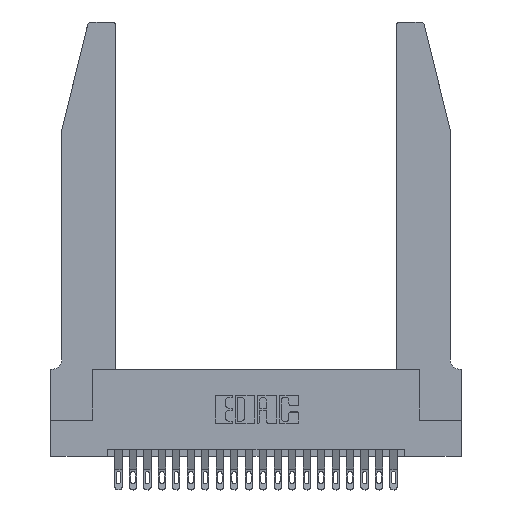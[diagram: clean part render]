
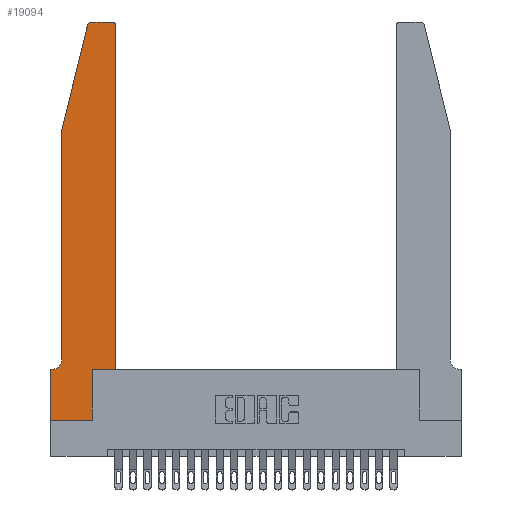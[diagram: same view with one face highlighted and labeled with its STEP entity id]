
A CAD part, top view. The second image highlights one B-rep face of the part: STEP entity #19094.
In plain terms, the highlighted planar face has unit normal (0, 0, 1).
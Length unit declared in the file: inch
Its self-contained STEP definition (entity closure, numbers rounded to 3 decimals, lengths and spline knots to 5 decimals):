
#271 = EDGE_CURVE ( 'NONE', #17309, #3389, #23285, .T. ) ;
#489 = CIRCLE ( 'NONE', #20541, 0.03 ) ;
#499 = DIRECTION ( 'NONE',  ( -0.239, -0.971, 0. ) ) ;
#606 = CARTESIAN_POINT ( 'NONE',  ( 0.4205, 2.72, 0.37 ) ) ;
#1068 = AXIS2_PLACEMENT_3D ( 'NONE', #5403, #18221, #7333 ) ;
#1088 = EDGE_CURVE ( 'NONE', #18876, #5038, #19748, .T. ) ;
#1273 = DIRECTION ( 'NONE',  ( 1., 0., 0. ) ) ;
#1359 = DIRECTION ( 'NONE',  ( 0., -1., 0. ) ) ;
#1726 = VERTEX_POINT ( 'NONE', #6758 ) ;
#1864 = CARTESIAN_POINT ( 'NONE',  ( 0.25487, 2.72718, 0.37 ) ) ;
#1869 = VECTOR ( 'NONE', #23675, 39.37008 ) ;
#1931 = EDGE_CURVE ( 'NONE', #5723, #22449, #6940, .T. ) ;
#2140 = ORIENTED_EDGE ( 'NONE', *, *, #1088, .T. ) ;
#2168 = VERTEX_POINT ( 'NONE', #3895 ) ;
#2270 = CARTESIAN_POINT ( 'NONE',  ( 0., 0.35, 0.37 ) ) ;
#2541 = DIRECTION ( 'NONE',  ( 1., 0., 0. ) ) ;
#2691 = EDGE_CURVE ( 'NONE', #18777, #18876, #12182, .T. ) ;
#3153 = CIRCLE ( 'NONE', #1068, 0.07 ) ;
#3180 = PLANE ( 'NONE',  #20446 ) ;
#3389 = VERTEX_POINT ( 'NONE', #19298 ) ;
#3895 = CARTESIAN_POINT ( 'NONE',  ( 0.0055, 0.35, 0.37 ) ) ;
#4066 = CARTESIAN_POINT ( 'NONE',  ( 0.4205, 2.75, 0.37 ) ) ;
#4377 = CARTESIAN_POINT ( 'NONE',  ( 0.0755, 2., 0.37 ) ) ;
#4488 = VERTEX_POINT ( 'NONE', #22270 ) ;
#4607 = EDGE_CURVE ( 'NONE', #21902, #5723, #18485, .T. ) ;
#4656 = VECTOR ( 'NONE', #5742, 39.37008 ) ;
#5038 = VERTEX_POINT ( 'NONE', #21862 ) ;
#5403 = CARTESIAN_POINT ( 'NONE',  ( 0.0055, 0.42, 0.37 ) ) ;
#5723 = VERTEX_POINT ( 'NONE', #9866 ) ;
#5742 = DIRECTION ( 'NONE',  ( 0., 1., 0. ) ) ;
#5915 = ORIENTED_EDGE ( 'NONE', *, *, #11713, .T. ) ;
#6308 = ORIENTED_EDGE ( 'NONE', *, *, #20932, .T. ) ;
#6758 = CARTESIAN_POINT ( 'NONE',  ( 0.2865, 0.35, 0.37 ) ) ;
#6940 = LINE ( 'NONE', #14252, #1869 ) ;
#7024 = CARTESIAN_POINT ( 'NONE',  ( 0., 0.35, 0.37 ) ) ;
#7093 = CARTESIAN_POINT ( 'NONE',  ( 0.2605, 2.75, 0.37 ) ) ;
#7333 = DIRECTION ( 'NONE',  ( -1., 0., 0. ) ) ;
#7954 = VERTEX_POINT ( 'NONE', #11986 ) ;
#7981 = EDGE_CURVE ( 'NONE', #7954, #4488, #15835, .T. ) ;
#8278 = VECTOR ( 'NONE', #499, 39.37008 ) ;
#8295 = DIRECTION ( 'NONE',  ( 0., 1., 0. ) ) ;
#9137 = CIRCLE ( 'NONE', #20680, 0.03 ) ;
#9436 = EDGE_LOOP ( 'NONE', ( #10798, #17330, #14394, #10636, #5915, #6308, #18889, #2140, #14486, #20805, #21057, #19264 ) ) ;
#9866 = CARTESIAN_POINT ( 'NONE',  ( 0.0755, 2., 0.37 ) ) ;
#10212 = VECTOR ( 'NONE', #17427, 39.37008 ) ;
#10486 = LINE ( 'NONE', #14437, #18902 ) ;
#10636 = ORIENTED_EDGE ( 'NONE', *, *, #1931, .T. ) ;
#10798 = ORIENTED_EDGE ( 'NONE', *, *, #271, .T. ) ;
#11656 = CARTESIAN_POINT ( 'NONE',  ( 0., 0., 0.37 ) ) ;
#11713 = EDGE_CURVE ( 'NONE', #22449, #2168, #3153, .T. ) ;
#11849 = EDGE_CURVE ( 'NONE', #5038, #1726, #19782, .T. ) ;
#11914 = CARTESIAN_POINT ( 'NONE',  ( 0.0755, 0.35, 0.37 ) ) ;
#11986 = CARTESIAN_POINT ( 'NONE',  ( 0.4505, 0.35, 0.37 ) ) ;
#12066 = CARTESIAN_POINT ( 'NONE',  ( 0.4505, 0.35, 0.37 ) ) ;
#12182 = LINE ( 'NONE', #11656, #21630 ) ;
#12587 = DIRECTION ( 'NONE',  ( 0., 0., 1. ) ) ;
#12662 = DIRECTION ( 'NONE',  ( 1., 0., 0. ) ) ;
#13810 = DIRECTION ( 'NONE',  ( 0., 0., 1. ) ) ;
#13813 = EDGE_CURVE ( 'NONE', #1726, #7954, #10486, .T. ) ;
#14252 = CARTESIAN_POINT ( 'NONE',  ( 0.0755, 2., 0.37 ) ) ;
#14394 = ORIENTED_EDGE ( 'NONE', *, *, #4607, .T. ) ;
#14437 = CARTESIAN_POINT ( 'NONE',  ( 0.4505, 0.35, 0.37 ) ) ;
#14486 = ORIENTED_EDGE ( 'NONE', *, *, #11849, .T. ) ;
#15489 = EDGE_CURVE ( 'NONE', #4488, #17309, #9137, .T. ) ;
#15835 = LINE ( 'NONE', #12066, #19945 ) ;
#16370 = EDGE_CURVE ( 'NONE', #3389, #21902, #489, .T. ) ;
#17059 = CARTESIAN_POINT ( 'NONE',  ( 0., 0., 0.37 ) ) ;
#17309 = VERTEX_POINT ( 'NONE', #4066 ) ;
#17330 = ORIENTED_EDGE ( 'NONE', *, *, #16370, .T. ) ;
#17427 = DIRECTION ( 'NONE',  ( 1., 0., 0. ) ) ;
#18060 = DIRECTION ( 'NONE',  ( 1., 0., 0. ) ) ;
#18070 = VECTOR ( 'NONE', #18490, 39.37008 ) ;
#18221 = DIRECTION ( 'NONE',  ( 0., 0., -1. ) ) ;
#18485 = LINE ( 'NONE', #4377, #8278 ) ;
#18490 = DIRECTION ( 'NONE',  ( -1., 0., 0. ) ) ;
#18517 = VECTOR ( 'NONE', #19056, 39.37008 ) ;
#18777 = VERTEX_POINT ( 'NONE', #2270 ) ;
#18876 = VERTEX_POINT ( 'NONE', #19088 ) ;
#18889 = ORIENTED_EDGE ( 'NONE', *, *, #2691, .T. ) ;
#18902 = VECTOR ( 'NONE', #18060, 39.37008 ) ;
#19056 = DIRECTION ( 'NONE',  ( -1., 0., 0. ) ) ;
#19074 = LINE ( 'NONE', #11914, #18517 ) ;
#19088 = CARTESIAN_POINT ( 'NONE',  ( 0., 0., 0.37 ) ) ;
#19094 = ADVANCED_FACE ( 'NONE', ( #21665 ), #3180, .T. ) ;
#19264 = ORIENTED_EDGE ( 'NONE', *, *, #15489, .T. ) ;
#19298 = CARTESIAN_POINT ( 'NONE',  ( 0.284, 2.75, 0.37 ) ) ;
#19748 = LINE ( 'NONE', #17059, #10212 ) ;
#19782 = LINE ( 'NONE', #22071, #4656 ) ;
#19840 = CARTESIAN_POINT ( 'NONE',  ( 0.0755, 0.42, 0.37 ) ) ;
#19945 = VECTOR ( 'NONE', #8295, 39.37008 ) ;
#20446 = AXIS2_PLACEMENT_3D ( 'NONE', #7024, #23233, #12662 ) ;
#20541 = AXIS2_PLACEMENT_3D ( 'NONE', #23164, #12587, #1273 ) ;
#20680 = AXIS2_PLACEMENT_3D ( 'NONE', #606, #13810, #2541 ) ;
#20805 = ORIENTED_EDGE ( 'NONE', *, *, #13813, .T. ) ;
#20932 = EDGE_CURVE ( 'NONE', #2168, #18777, #19074, .T. ) ;
#21057 = ORIENTED_EDGE ( 'NONE', *, *, #7981, .T. ) ;
#21630 = VECTOR ( 'NONE', #1359, 39.37008 ) ;
#21665 = FACE_OUTER_BOUND ( 'NONE', #9436, .T. ) ;
#21862 = CARTESIAN_POINT ( 'NONE',  ( 0.2865, 0., 0.37 ) ) ;
#21902 = VERTEX_POINT ( 'NONE', #1864 ) ;
#22071 = CARTESIAN_POINT ( 'NONE',  ( 0.2865, 0.35, 0.37 ) ) ;
#22270 = CARTESIAN_POINT ( 'NONE',  ( 0.4505, 2.72, 0.37 ) ) ;
#22449 = VERTEX_POINT ( 'NONE', #19840 ) ;
#23164 = CARTESIAN_POINT ( 'NONE',  ( 0.284, 2.72, 0.37 ) ) ;
#23233 = DIRECTION ( 'NONE',  ( 0., 0., 1. ) ) ;
#23285 = LINE ( 'NONE', #7093, #18070 ) ;
#23675 = DIRECTION ( 'NONE',  ( 0., -1., 0. ) ) ;
